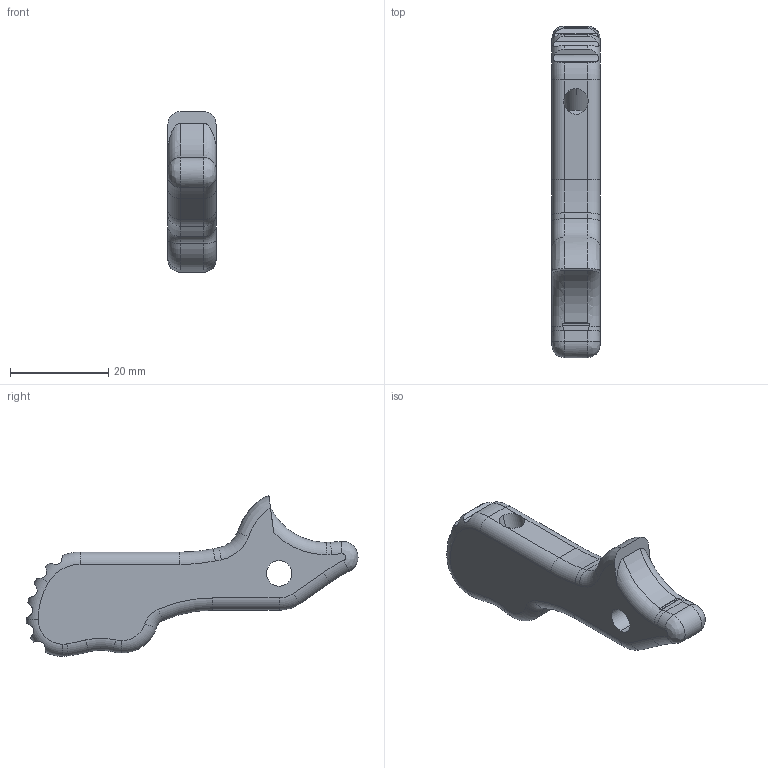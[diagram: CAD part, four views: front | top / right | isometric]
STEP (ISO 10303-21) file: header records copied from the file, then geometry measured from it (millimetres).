
FILE_DESCRIPTION (( 'STEP AP214' ), '1' );
FILE_NAME ('Hammer_.22_LR.STEP', '2014-02-22T02:15:11', ( '' ), ( '' ), 'SwSTEP 2.0', 'SolidWorks 2013', '' );
FILE_SCHEMA (( 'AUTOMOTIVE_DESIGN' ));
Length unit declared in the file: millimetre
Products named in the file (1): Hammer_.22_LR
Bounding box: 9.8 x 67.74 x 32.83 mm (x, y, z)
Volume: 9349.4 mm3; surface area: 3764.8 mm2
Topology: 1 solids, 1 shells, 106 faces, 272 edges, 168 vertices
Faces by surface type: cylinder 46, torus 32, plane 22, bspline 6
Entity records: 3960 total; most frequent: CARTESIAN_POINT 1431, ORIENTED_EDGE 544, DIRECTION 520, EDGE_CURVE 272, AXIS2_PLACEMENT_3D 221, VERTEX_POINT 168, CIRCLE 120, EDGE_LOOP 108
